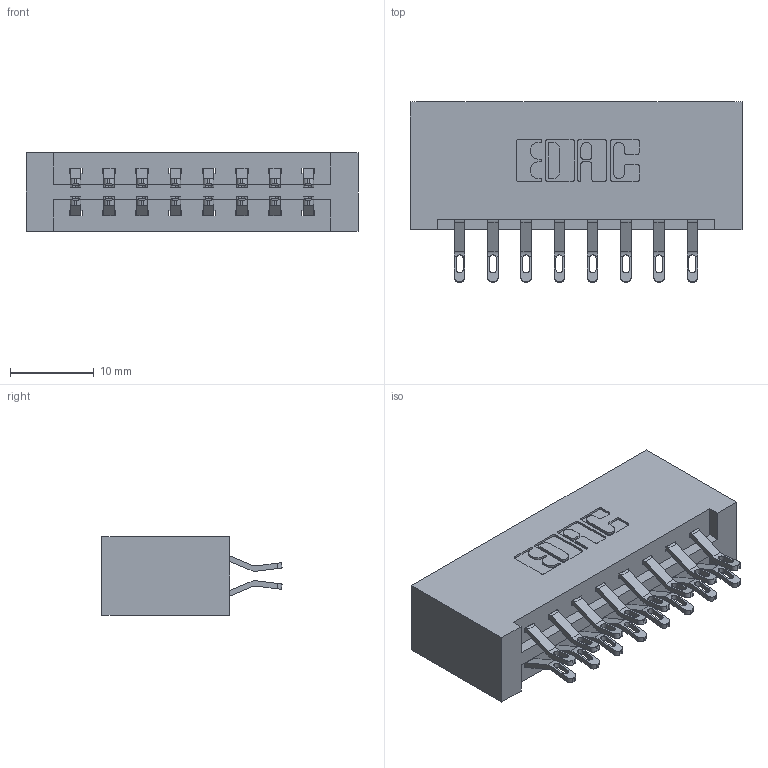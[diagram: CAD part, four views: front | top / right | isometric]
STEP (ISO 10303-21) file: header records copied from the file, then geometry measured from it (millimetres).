
FILE_DESCRIPTION (( 'STEP AP203' ), '1' );
FILE_NAME ('337-016-555-201.STEP', '2018-08-04T20:09:12', ( '' ), ( '' ), 'SwSTEP 2.0', 'SolidWorks 2016', '' );
FILE_SCHEMA (( 'CONFIG_CONTROL_DESIGN' ));
Length unit declared in the file: inch
Products named in the file (3): 337 Part_No Mounting Lugs; 345-292-001_555 Tail; 337-016-555-201
Assembly tree (17 placements, depth 2):
  337-016-555-201
    337 Part_No Mounting Lugs
    345-292-001_555 Tail  x16
Bounding box: 39.57 x 21.47 x 9.4 mm (x, y, z)
Volume: 4525.1 mm3; surface area: 5016.4 mm2
Topology: 17 solids, 17 shells, 1066 faces, 3311 edges, 2206 vertices
Faces by surface type: plane 642, cylinder 424
Entity records: 10649 total; most frequent: CARTESIAN_POINT 1856, ORIENTED_EDGE 1762, DIRECTION 1605, EDGE_CURVE 881, LINE 741, VECTOR 741, VERTEX_POINT 586, AXIS2_PLACEMENT_3D 432
